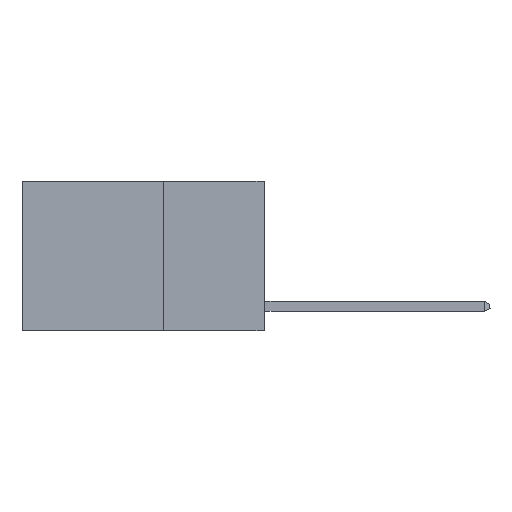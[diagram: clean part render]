
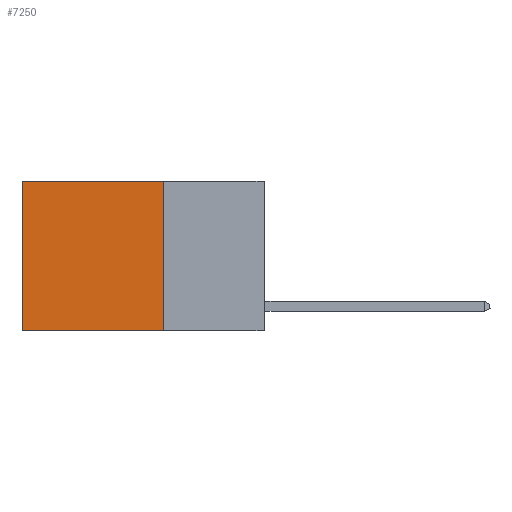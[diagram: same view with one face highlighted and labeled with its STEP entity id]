
A CAD part, left-side view. The second image highlights one B-rep face of the part: STEP entity #7250.
In plain terms, the highlighted planar face has unit normal (-1, 0, 0).
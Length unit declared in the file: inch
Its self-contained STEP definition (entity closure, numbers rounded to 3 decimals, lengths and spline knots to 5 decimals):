
#51 = FACE_OUTER_BOUND ( 'NONE', #10725, .T. ) ;
#494 = CARTESIAN_POINT ( 'NONE',  ( 0.2625, 0.25, 0. ) ) ;
#602 = DIRECTION ( 'NONE',  ( 0., 1., 0. ) ) ;
#1276 = CARTESIAN_POINT ( 'NONE',  ( 0.2625, 0.25, 0. ) ) ;
#2318 = LINE ( 'NONE', #4704, #8652 ) ;
#2518 = VERTEX_POINT ( 'NONE', #494 ) ;
#3055 = LINE ( 'NONE', #4539, #6026 ) ;
#3356 = CARTESIAN_POINT ( 'NONE',  ( 0.2625, 0.6, 0. ) ) ;
#4409 = CARTESIAN_POINT ( 'NONE',  ( 0.2625, 0.25, 0. ) ) ;
#4539 = CARTESIAN_POINT ( 'NONE',  ( 0.2625, 0.25, -0.37 ) ) ;
#4704 = CARTESIAN_POINT ( 'NONE',  ( 0.2625, 0.6, 0. ) ) ;
#4868 = ORIENTED_EDGE ( 'NONE', *, *, #12550, .F. ) ;
#5060 = VECTOR ( 'NONE', #10678, 39.37008 ) ;
#5119 = VERTEX_POINT ( 'NONE', #9802 ) ;
#5434 = AXIS2_PLACEMENT_3D ( 'NONE', #1276, #15096, #6227 ) ;
#5650 = LINE ( 'NONE', #4409, #5060 ) ;
#5848 = EDGE_CURVE ( 'NONE', #2518, #5119, #14578, .T. ) ;
#6026 = VECTOR ( 'NONE', #602, 39.37008 ) ;
#6227 = DIRECTION ( 'NONE',  ( 0., 0., -1. ) ) ;
#6311 = PLANE ( 'NONE',  #5434 ) ;
#6435 = VECTOR ( 'NONE', #13845, 39.37008 ) ;
#6846 = ORIENTED_EDGE ( 'NONE', *, *, #5848, .F. ) ;
#7250 = ADVANCED_FACE ( 'NONE', ( #51 ), #6311, .F. ) ;
#7348 = DIRECTION ( 'NONE',  ( 0., 0., -1. ) ) ;
#8652 = VECTOR ( 'NONE', #7348, 39.37008 ) ;
#8940 = CARTESIAN_POINT ( 'NONE',  ( 0.2625, 0.25, 0. ) ) ;
#9802 = CARTESIAN_POINT ( 'NONE',  ( 0.2625, 0.25, -0.37 ) ) ;
#10474 = VERTEX_POINT ( 'NONE', #11860 ) ;
#10678 = DIRECTION ( 'NONE',  ( 0., 1., 0. ) ) ;
#10725 = EDGE_LOOP ( 'NONE', ( #13913, #4868, #6846, #14194 ) ) ;
#11355 = VERTEX_POINT ( 'NONE', #3356 ) ;
#11860 = CARTESIAN_POINT ( 'NONE',  ( 0.2625, 0.6, -0.37 ) ) ;
#12550 = EDGE_CURVE ( 'NONE', #5119, #10474, #3055, .T. ) ;
#12753 = EDGE_CURVE ( 'NONE', #11355, #10474, #2318, .T. ) ;
#13845 = DIRECTION ( 'NONE',  ( 0., 0., -1. ) ) ;
#13913 = ORIENTED_EDGE ( 'NONE', *, *, #12753, .T. ) ;
#14194 = ORIENTED_EDGE ( 'NONE', *, *, #15304, .T. ) ;
#14578 = LINE ( 'NONE', #8940, #6435 ) ;
#15096 = DIRECTION ( 'NONE',  ( 1., 0., 0. ) ) ;
#15304 = EDGE_CURVE ( 'NONE', #2518, #11355, #5650, .T. ) ;
